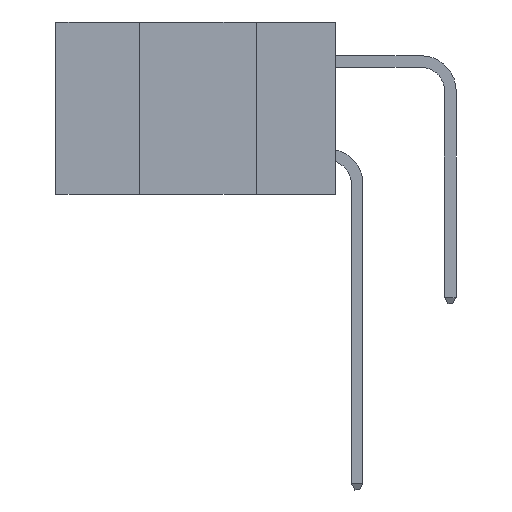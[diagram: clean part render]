
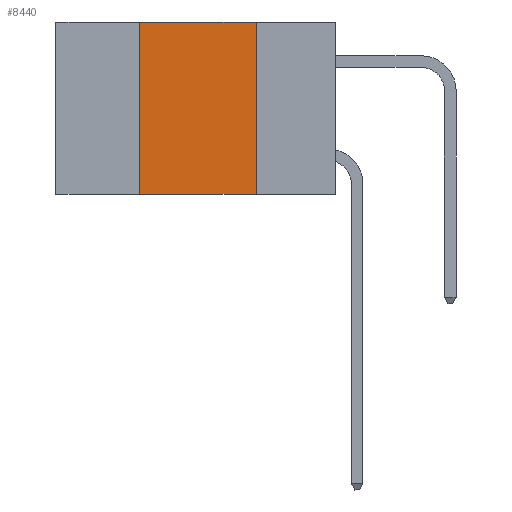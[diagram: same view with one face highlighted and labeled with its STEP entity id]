
A CAD part, left-side view. The second image highlights one B-rep face of the part: STEP entity #8440.
In plain terms, the highlighted planar face has unit normal (-1, 0, 0).
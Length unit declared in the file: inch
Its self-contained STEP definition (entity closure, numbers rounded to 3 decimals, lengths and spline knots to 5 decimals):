
#940 = DIRECTION ( 'NONE',  ( 0., 0., -1. ) ) ;
#1023 = ORIENTED_EDGE ( 'NONE', *, *, #10694, .F. ) ;
#1639 = CARTESIAN_POINT ( 'NONE',  ( 0., 0.17, 0. ) ) ;
#2231 = VERTEX_POINT ( 'NONE', #9656 ) ;
#2502 = ORIENTED_EDGE ( 'NONE', *, *, #2910, .F. ) ;
#2774 = CARTESIAN_POINT ( 'NONE',  ( 0., 0.6, -0.37 ) ) ;
#2878 = VERTEX_POINT ( 'NONE', #16636 ) ;
#2910 = EDGE_CURVE ( 'NONE', #15185, #2231, #8468, .T. ) ;
#3010 = VERTEX_POINT ( 'NONE', #4664 ) ;
#3311 = LINE ( 'NONE', #14794, #13347 ) ;
#4263 = CARTESIAN_POINT ( 'NONE',  ( 0., 0.6, 0. ) ) ;
#4429 = DIRECTION ( 'NONE',  ( 0., 0., -1. ) ) ;
#4664 = CARTESIAN_POINT ( 'NONE',  ( 0., 0.42, -0.37 ) ) ;
#4765 = ORIENTED_EDGE ( 'NONE', *, *, #14407, .F. ) ;
#5355 = EDGE_CURVE ( 'NONE', #3010, #2231, #13306, .T. ) ;
#5895 = VECTOR ( 'NONE', #4429, 39.37008 ) ;
#6041 = VECTOR ( 'NONE', #15125, 39.37008 ) ;
#6647 = FACE_OUTER_BOUND ( 'NONE', #14166, .T. ) ;
#7008 = DIRECTION ( 'NONE',  ( 0., -1., 0. ) ) ;
#8296 = VECTOR ( 'NONE', #7008, 39.37008 ) ;
#8440 = ADVANCED_FACE ( 'NONE', ( #6647 ), #10455, .F. ) ;
#8468 = LINE ( 'NONE', #1639, #5895 ) ;
#9016 = DIRECTION ( 'NONE',  ( 1., 0., 0. ) ) ;
#9656 = CARTESIAN_POINT ( 'NONE',  ( 0., 0.17, -0.37 ) ) ;
#10455 = PLANE ( 'NONE',  #12445 ) ;
#10694 = EDGE_CURVE ( 'NONE', #2878, #15185, #17306, .T. ) ;
#10975 = DIRECTION ( 'NONE',  ( 0., 0., 1. ) ) ;
#12429 = CARTESIAN_POINT ( 'NONE',  ( 0., 0.17, 0. ) ) ;
#12445 = AXIS2_PLACEMENT_3D ( 'NONE', #17344, #9016, #940 ) ;
#12801 = ORIENTED_EDGE ( 'NONE', *, *, #5355, .T. ) ;
#13306 = LINE ( 'NONE', #2774, #6041 ) ;
#13347 = VECTOR ( 'NONE', #10975, 39.37008 ) ;
#14166 = EDGE_LOOP ( 'NONE', ( #2502, #1023, #4765, #12801 ) ) ;
#14407 = EDGE_CURVE ( 'NONE', #3010, #2878, #3311, .T. ) ;
#14794 = CARTESIAN_POINT ( 'NONE',  ( 0., 0.42, 0. ) ) ;
#15125 = DIRECTION ( 'NONE',  ( 0., -1., 0. ) ) ;
#15185 = VERTEX_POINT ( 'NONE', #12429 ) ;
#16636 = CARTESIAN_POINT ( 'NONE',  ( 0., 0.42, 0. ) ) ;
#17306 = LINE ( 'NONE', #4263, #8296 ) ;
#17344 = CARTESIAN_POINT ( 'NONE',  ( 0., 0.6, 0. ) ) ;
